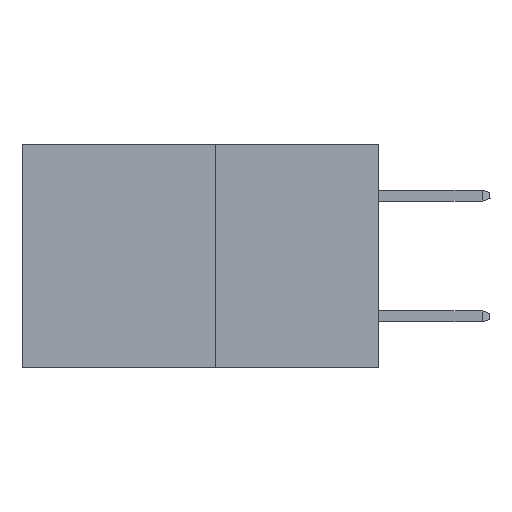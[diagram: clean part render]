
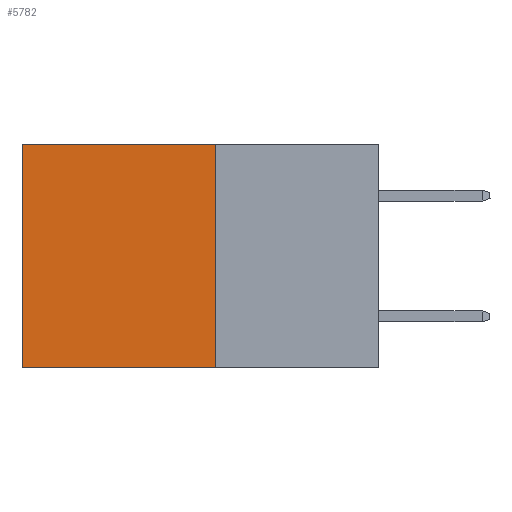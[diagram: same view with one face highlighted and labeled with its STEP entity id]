
A CAD part, left-side view. The second image highlights one B-rep face of the part: STEP entity #5782.
In plain terms, the highlighted planar face has unit normal (-1, 0, 0).
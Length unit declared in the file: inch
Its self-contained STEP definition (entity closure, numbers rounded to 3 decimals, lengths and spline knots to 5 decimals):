
#70 = VERTEX_POINT ( 'NONE', #2887 ) ;
#401 = ORIENTED_EDGE ( 'NONE', *, *, #8243, .F. ) ;
#481 = FACE_OUTER_BOUND ( 'NONE', #3095, .T. ) ;
#633 = VECTOR ( 'NONE', #5497, 39.37008 ) ;
#841 = AXIS2_PLACEMENT_3D ( 'NONE', #6195, #5495, #5461 ) ;
#982 = VECTOR ( 'NONE', #6110, 39.37008 ) ;
#1184 = ORIENTED_EDGE ( 'NONE', *, *, #5354, .T. ) ;
#1407 = CARTESIAN_POINT ( 'NONE',  ( 0.277, 0.27, -0.37 ) ) ;
#1430 = VECTOR ( 'NONE', #7823, 39.37008 ) ;
#1538 = CARTESIAN_POINT ( 'NONE',  ( 0.277, 0.59, -0.37 ) ) ;
#1585 = ORIENTED_EDGE ( 'NONE', *, *, #6138, .F. ) ;
#1713 = ORIENTED_EDGE ( 'NONE', *, *, #4827, .T. ) ;
#2412 = VECTOR ( 'NONE', #7463, 39.37008 ) ;
#2564 = LINE ( 'NONE', #1407, #982 ) ;
#2887 = CARTESIAN_POINT ( 'NONE',  ( 0.277, 0.27, 0. ) ) ;
#3095 = EDGE_LOOP ( 'NONE', ( #1713, #1585, #401, #1184 ) ) ;
#3286 = VERTEX_POINT ( 'NONE', #6261 ) ;
#3441 = PLANE ( 'NONE',  #841 ) ;
#3667 = CARTESIAN_POINT ( 'NONE',  ( 0.277, 0.27, -0.37 ) ) ;
#3974 = LINE ( 'NONE', #1538, #633 ) ;
#4272 = VERTEX_POINT ( 'NONE', #5947 ) ;
#4827 = EDGE_CURVE ( 'NONE', #5521, #3286, #3974, .T. ) ;
#5299 = CARTESIAN_POINT ( 'NONE',  ( 0.277, 0.27, 0. ) ) ;
#5354 = EDGE_CURVE ( 'NONE', #70, #5521, #6166, .T. ) ;
#5461 = DIRECTION ( 'NONE',  ( 0., 0., -1. ) ) ;
#5495 = DIRECTION ( 'NONE',  ( 1., 0., 0. ) ) ;
#5497 = DIRECTION ( 'NONE',  ( 0., 0., -1. ) ) ;
#5521 = VERTEX_POINT ( 'NONE', #6397 ) ;
#5782 = ADVANCED_FACE ( 'NONE', ( #481 ), #3441, .F. ) ;
#5947 = CARTESIAN_POINT ( 'NONE',  ( 0.277, 0.27, -0.37 ) ) ;
#6110 = DIRECTION ( 'NONE',  ( 0., 0., -1. ) ) ;
#6138 = EDGE_CURVE ( 'NONE', #4272, #3286, #6638, .T. ) ;
#6166 = LINE ( 'NONE', #5299, #2412 ) ;
#6195 = CARTESIAN_POINT ( 'NONE',  ( 0.277, 0.27, -0.37 ) ) ;
#6261 = CARTESIAN_POINT ( 'NONE',  ( 0.277, 0.59, -0.37 ) ) ;
#6397 = CARTESIAN_POINT ( 'NONE',  ( 0.277, 0.59, 0. ) ) ;
#6638 = LINE ( 'NONE', #3667, #1430 ) ;
#7463 = DIRECTION ( 'NONE',  ( 0., 1., 0. ) ) ;
#7823 = DIRECTION ( 'NONE',  ( 0., 1., 0. ) ) ;
#8243 = EDGE_CURVE ( 'NONE', #70, #4272, #2564, .T. ) ;
